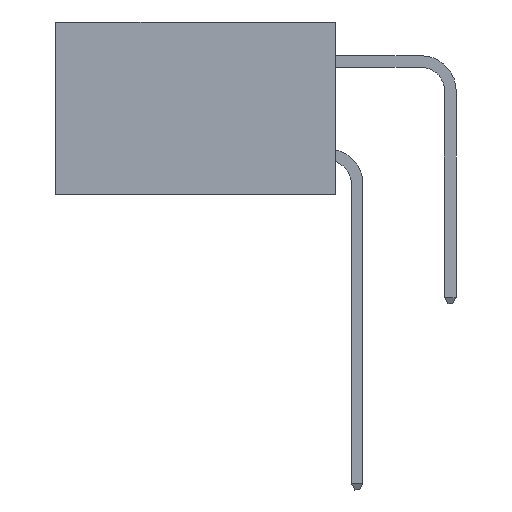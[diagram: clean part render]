
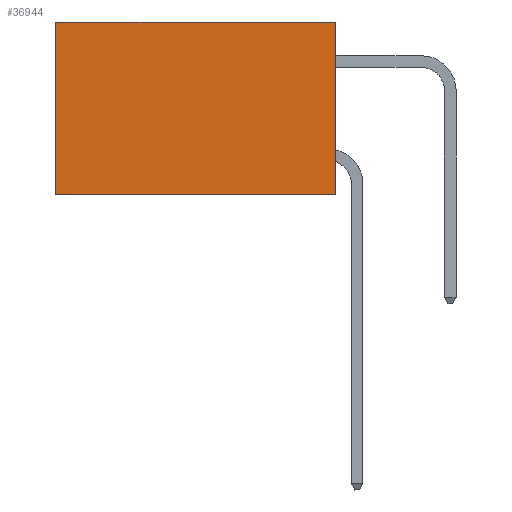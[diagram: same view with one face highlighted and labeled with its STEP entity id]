
A CAD part, left-side view. The second image highlights one B-rep face of the part: STEP entity #36944.
In plain terms, the highlighted planar face has unit normal (-1, 0, 0).
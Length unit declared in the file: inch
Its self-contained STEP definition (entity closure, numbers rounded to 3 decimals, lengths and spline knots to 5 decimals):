
#504 = ORIENTED_EDGE ( 'NONE', *, *, #37083, .T. ) ;
#691 = DIRECTION ( 'NONE',  ( 0., 0., -1. ) ) ;
#3040 = VECTOR ( 'NONE', #25986, 39.37008 ) ;
#3216 = ORIENTED_EDGE ( 'NONE', *, *, #12503, .F. ) ;
#5040 = LINE ( 'NONE', #35331, #3040 ) ;
#5583 = LINE ( 'NONE', #37003, #29385 ) ;
#6395 = LINE ( 'NONE', #16309, #21951 ) ;
#7657 = ORIENTED_EDGE ( 'NONE', *, *, #36612, .F. ) ;
#7797 = CARTESIAN_POINT ( 'NONE',  ( 0.2875, 0., 0. ) ) ;
#7848 = CARTESIAN_POINT ( 'NONE',  ( 0.2875, 0., 0. ) ) ;
#8458 = EDGE_CURVE ( 'NONE', #13348, #33921, #5040, .T. ) ;
#9034 = DIRECTION ( 'NONE',  ( 0., 1., 0. ) ) ;
#9418 = CARTESIAN_POINT ( 'NONE',  ( 0.2875, 0.6, 0. ) ) ;
#10936 = DIRECTION ( 'NONE',  ( 0., 0., -1. ) ) ;
#10938 = CARTESIAN_POINT ( 'NONE',  ( 0.2875, 0.6, -0.37 ) ) ;
#11007 = ORIENTED_EDGE ( 'NONE', *, *, #8458, .T. ) ;
#11434 = AXIS2_PLACEMENT_3D ( 'NONE', #7797, #29507, #10936 ) ;
#12503 = EDGE_CURVE ( 'NONE', #13348, #37738, #6395, .T. ) ;
#13348 = VERTEX_POINT ( 'NONE', #7848 ) ;
#13973 = LINE ( 'NONE', #30756, #30392 ) ;
#16309 = CARTESIAN_POINT ( 'NONE',  ( 0.2875, 0., 0. ) ) ;
#21951 = VECTOR ( 'NONE', #691, 39.37008 ) ;
#22353 = CARTESIAN_POINT ( 'NONE',  ( 0.2875, 0., -0.37 ) ) ;
#24600 = EDGE_LOOP ( 'NONE', ( #504, #7657, #3216, #11007 ) ) ;
#25986 = DIRECTION ( 'NONE',  ( 0., 1., 0. ) ) ;
#26007 = FACE_OUTER_BOUND ( 'NONE', #24600, .T. ) ;
#29385 = VECTOR ( 'NONE', #37128, 39.37008 ) ;
#29507 = DIRECTION ( 'NONE',  ( 1., 0., 0. ) ) ;
#30392 = VECTOR ( 'NONE', #9034, 39.37008 ) ;
#30756 = CARTESIAN_POINT ( 'NONE',  ( 0.2875, 0., -0.37 ) ) ;
#33687 = VERTEX_POINT ( 'NONE', #10938 ) ;
#33921 = VERTEX_POINT ( 'NONE', #9418 ) ;
#35331 = CARTESIAN_POINT ( 'NONE',  ( 0.2875, 0., 0. ) ) ;
#36612 = EDGE_CURVE ( 'NONE', #37738, #33687, #13973, .T. ) ;
#36944 = ADVANCED_FACE ( 'NONE', ( #26007 ), #38669, .F. ) ;
#37003 = CARTESIAN_POINT ( 'NONE',  ( 0.2875, 0.6, 0. ) ) ;
#37083 = EDGE_CURVE ( 'NONE', #33921, #33687, #5583, .T. ) ;
#37128 = DIRECTION ( 'NONE',  ( 0., 0., -1. ) ) ;
#37738 = VERTEX_POINT ( 'NONE', #22353 ) ;
#38669 = PLANE ( 'NONE',  #11434 ) ;
